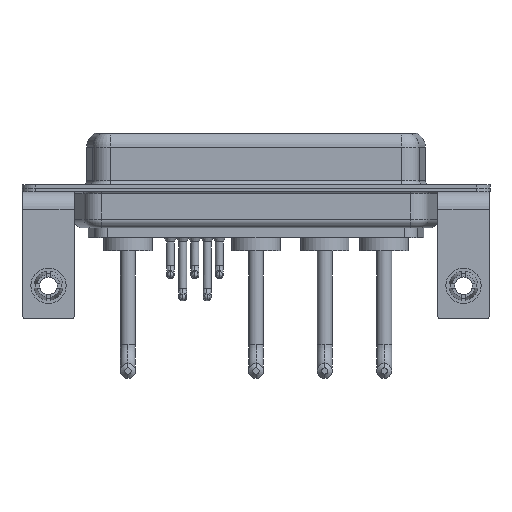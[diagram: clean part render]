
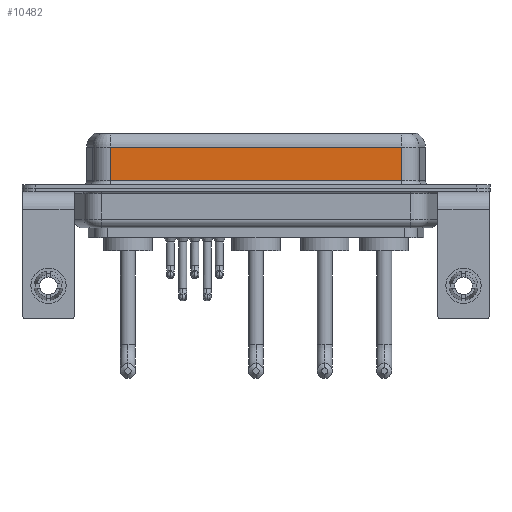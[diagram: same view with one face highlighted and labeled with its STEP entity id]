
A CAD part, front view. The second image highlights one B-rep face of the part: STEP entity #10482.
In plain terms, the highlighted planar face has unit normal (0, -1, 0).
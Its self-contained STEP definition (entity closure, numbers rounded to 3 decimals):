
#538 = DIRECTION ( 'NONE',  ( 0., 0., -1. ) ) ;
#1014 = CARTESIAN_POINT ( 'NONE',  ( 7.013, -3.95, 6.4 ) ) ;
#1404 = CARTESIAN_POINT ( 'NONE',  ( 40.037, -3.95, 0.9 ) ) ;
#2665 = EDGE_CURVE ( 'NONE', #10456, #6927, #19465, .T. ) ;
#2856 = CARTESIAN_POINT ( 'NONE',  ( 40.037, -3.95, 6.4 ) ) ;
#3145 = DIRECTION ( 'NONE',  ( 0., 0., 1. ) ) ;
#3255 = VECTOR ( 'NONE', #17664, 1000. ) ;
#4234 = VECTOR ( 'NONE', #538, 1000. ) ;
#5140 = CARTESIAN_POINT ( 'NONE',  ( 40.037, -3.95, 6.4 ) ) ;
#5305 = ORIENTED_EDGE ( 'NONE', *, *, #13379, .T. ) ;
#6129 = DIRECTION ( 'NONE',  ( 0., 1., 0. ) ) ;
#6217 = VERTEX_POINT ( 'NONE', #9599 ) ;
#6802 = VECTOR ( 'NONE', #13329, 1000. ) ;
#6927 = VERTEX_POINT ( 'NONE', #13169 ) ;
#7657 = DIRECTION ( 'NONE',  ( 1., 0., 0. ) ) ;
#8072 = VERTEX_POINT ( 'NONE', #15427 ) ;
#8555 = VECTOR ( 'NONE', #7657, 1000. ) ;
#8557 = CARTESIAN_POINT ( 'NONE',  ( 40.037, -3.95, 4.65 ) ) ;
#8580 = EDGE_LOOP ( 'NONE', ( #15568, #18539, #5305, #12233 ) ) ;
#8774 = LINE ( 'NONE', #1014, #6802 ) ;
#9599 = CARTESIAN_POINT ( 'NONE',  ( 40.037, -3.95, 0.9 ) ) ;
#10310 = FACE_OUTER_BOUND ( 'NONE', #8580, .T. ) ;
#10456 = VERTEX_POINT ( 'NONE', #17923 ) ;
#10482 = ADVANCED_FACE ( 'NONE', ( #10310 ), #17821, .F. ) ;
#12233 = ORIENTED_EDGE ( 'NONE', *, *, #16984, .T. ) ;
#12677 = EDGE_CURVE ( 'NONE', #10456, #6217, #14256, .T. ) ;
#13169 = CARTESIAN_POINT ( 'NONE',  ( 7.013, -3.95, 4.65 ) ) ;
#13329 = DIRECTION ( 'NONE',  ( 0., 0., -1. ) ) ;
#13379 = EDGE_CURVE ( 'NONE', #6927, #8072, #8774, .T. ) ;
#14256 = LINE ( 'NONE', #5140, #4234 ) ;
#14668 = AXIS2_PLACEMENT_3D ( 'NONE', #2856, #6129, #3145 ) ;
#15427 = CARTESIAN_POINT ( 'NONE',  ( 7.013, -3.95, 0.9 ) ) ;
#15568 = ORIENTED_EDGE ( 'NONE', *, *, #12677, .F. ) ;
#16984 = EDGE_CURVE ( 'NONE', #8072, #6217, #17970, .T. ) ;
#17664 = DIRECTION ( 'NONE',  ( -1., 0., 0. ) ) ;
#17821 = PLANE ( 'NONE',  #14668 ) ;
#17923 = CARTESIAN_POINT ( 'NONE',  ( 40.037, -3.95, 4.65 ) ) ;
#17970 = LINE ( 'NONE', #1404, #8555 ) ;
#18539 = ORIENTED_EDGE ( 'NONE', *, *, #2665, .T. ) ;
#19465 = LINE ( 'NONE', #8557, #3255 ) ;
